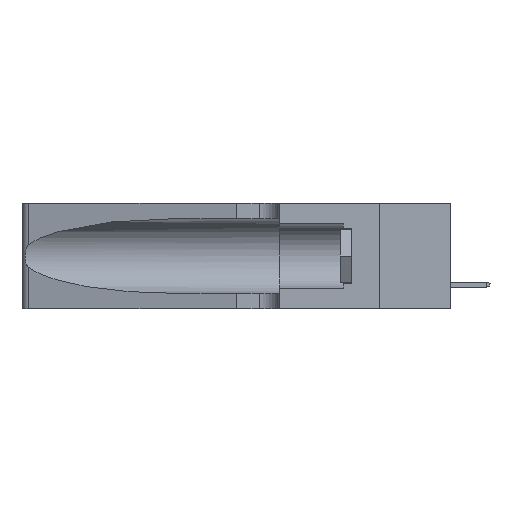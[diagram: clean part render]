
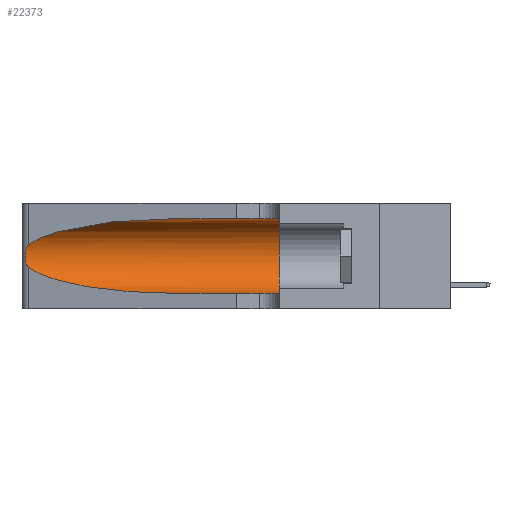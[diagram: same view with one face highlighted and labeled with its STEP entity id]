
A CAD part, left-side view. The second image highlights one B-rep face of the part: STEP entity #22373.
In plain terms, the highlighted cylindrical face has radius 3.308 mm (diameter 6.617 mm), a partial arc.
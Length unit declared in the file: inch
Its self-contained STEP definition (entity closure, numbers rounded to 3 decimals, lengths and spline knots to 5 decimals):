
#98 = VERTEX_POINT ( 'NONE', #26784 ) ;
#1078 = CARTESIAN_POINT ( 'NONE',  ( 0.18966, 0.96281, 0.31525 ) ) ;
#1134 = EDGE_CURVE ( 'NONE', #26663, #29288, #25005, .T. ) ;
#1286 = CARTESIAN_POINT ( 'NONE',  ( 0.26075, 1.23896, 0.19203 ) ) ;
#1718 = CARTESIAN_POINT ( 'NONE',  ( 0.1305, 1.61858, 0.31525 ) ) ;
#2033 =( BOUNDED_CURVE ( )  B_SPLINE_CURVE ( 3, ( #23238, #18377, #27946, #6050 ),
 .UNSPECIFIED., .F., .T. ) 
 B_SPLINE_CURVE_WITH_KNOTS ( ( 4, 4 ),
 ( 3.44316, 4.71239 ),
 .UNSPECIFIED. ) 
 CURVE ( )  GEOMETRIC_REPRESENTATION_ITEM ( )  RATIONAL_B_SPLINE_CURVE ( ( 1., 0.87, 0.87, 1. ) ) 
 REPRESENTATION_ITEM ( '' )  );
#2767 = ORIENTED_EDGE ( 'NONE', *, *, #27312, .F. ) ;
#2822 = CARTESIAN_POINT ( 'NONE',  ( 0.25487, 1.22718, 0.22369 ) ) ;
#3303 = DIRECTION ( 'NONE',  ( 0., 0., -1. ) ) ;
#3975 = DIRECTION ( 'NONE',  ( 0., -1., 0. ) ) ;
#4300 = CARTESIAN_POINT ( 'NONE',  ( 0.25487, 1.22718, 0.14631 ) ) ;
#5276 = CARTESIAN_POINT ( 'NONE',  ( 0.1305, 0.72297, 0.31525 ) ) ;
#5601 = CARTESIAN_POINT ( 'NONE',  ( 0.2373, 1.15595, 0.28018 ) ) ;
#5803 = CARTESIAN_POINT ( 'NONE',  ( 0.25487, 1.22718, 0.14631 ) ) ;
#6050 = CARTESIAN_POINT ( 'NONE',  ( 0.1305, 0.72297, 0.05475 ) ) ;
#6210 = DIRECTION ( 'NONE',  ( 0., 1., 0. ) ) ;
#7992 = DIRECTION ( 'NONE',  ( 0., -1., 0. ) ) ;
#8379 = VERTEX_POINT ( 'NONE', #13891 ) ;
#8678 = AXIS2_PLACEMENT_3D ( 'NONE', #25827, #6210, #30524 ) ;
#8873 = CARTESIAN_POINT ( 'NONE',  ( 0.26017, 1.23833, 0.17102 ) ) ;
#8969 = B_SPLINE_CURVE_WITH_KNOTS ( 'NONE', 3,
 ( #18126, #16009, #21191, #13913, #11004, #18280, #1286, #16162, #8873, #23297, #18605, #18762, #11482, #5803 ),
 .UNSPECIFIED., .F., .F.,
 ( 4, 2, 2, 2, 2, 2, 4 ),
 ( 0., 0.00027, 0.00053, 0.00107, 0.0016, 0.00187, 0.00214 ),
 .UNSPECIFIED. ) ;
#9220 = CIRCLE ( 'NONE', #8678, 0.13025 ) ;
#9975 = AXIS2_PLACEMENT_3D ( 'NONE', #25477, #7992, #3303 ) ;
#10598 = FACE_OUTER_BOUND ( 'NONE', #27418, .T. ) ;
#11004 = CARTESIAN_POINT ( 'NONE',  ( 0.25854, 1.2359, 0.20912 ) ) ;
#11482 = CARTESIAN_POINT ( 'NONE',  ( 0.25555, 1.22993, 0.14849 ) ) ;
#11602 = DIRECTION ( 'NONE',  ( 0., -1., 0. ) ) ;
#11761 = LINE ( 'NONE', #1718, #24561 ) ;
#13891 = CARTESIAN_POINT ( 'NONE',  ( 0.1305, 0.35, 0.05475 ) ) ;
#13913 = CARTESIAN_POINT ( 'NONE',  ( 0.25787, 1.23484, 0.2124 ) ) ;
#15491 = CARTESIAN_POINT ( 'NONE',  ( 0.25487, 1.22718, 0.22369 ) ) ;
#15577 = EDGE_CURVE ( 'NONE', #98, #8379, #9220, .T. ) ;
#16009 = CARTESIAN_POINT ( 'NONE',  ( 0.25555, 1.22994, 0.2215 ) ) ;
#16162 = CARTESIAN_POINT ( 'NONE',  ( 0.26075, 1.23896, 0.178 ) ) ;
#16557 = ORIENTED_EDGE ( 'NONE', *, *, #23697, .T. ) ;
#18126 = CARTESIAN_POINT ( 'NONE',  ( 0.25487, 1.22718, 0.22369 ) ) ;
#18280 = CARTESIAN_POINT ( 'NONE',  ( 0.26018, 1.23835, 0.19895 ) ) ;
#18377 = CARTESIAN_POINT ( 'NONE',  ( 0.2373, 1.15595, 0.08982 ) ) ;
#18458 = EDGE_CURVE ( 'NONE', #26011, #31255, #2033, .T. ) ;
#18605 = CARTESIAN_POINT ( 'NONE',  ( 0.25789, 1.23486, 0.15765 ) ) ;
#18762 = CARTESIAN_POINT ( 'NONE',  ( 0.25639, 1.23186, 0.15144 ) ) ;
#19315 = CARTESIAN_POINT ( 'NONE',  ( 0.1305, 0.72297, 0.31525 ) ) ;
#20826 = CARTESIAN_POINT ( 'NONE',  ( 0.1305, 1.61858, 0.05475 ) ) ;
#21191 = CARTESIAN_POINT ( 'NONE',  ( 0.25639, 1.23184, 0.21858 ) ) ;
#22373 = ADVANCED_FACE ( 'NONE', ( #10598 ), #30811, .F. ) ;
#23238 = CARTESIAN_POINT ( 'NONE',  ( 0.25487, 1.22718, 0.14631 ) ) ;
#23297 = CARTESIAN_POINT ( 'NONE',  ( 0.25856, 1.23593, 0.16098 ) ) ;
#23697 = EDGE_CURVE ( 'NONE', #31255, #8379, #26157, .T. ) ;
#24561 = VECTOR ( 'NONE', #11602, 39.37008 ) ;
#25005 =( BOUNDED_CURVE ( )  B_SPLINE_CURVE ( 3, ( #5276, #1078, #5601, #15491 ),
 .UNSPECIFIED., .F., .T. ) 
 B_SPLINE_CURVE_WITH_KNOTS ( ( 4, 4 ),
 ( 1.5708, 2.84003 ),
 .UNSPECIFIED. ) 
 CURVE ( )  GEOMETRIC_REPRESENTATION_ITEM ( )  RATIONAL_B_SPLINE_CURVE ( ( 1., 0.87, 0.87, 1. ) ) 
 REPRESENTATION_ITEM ( '' )  );
#25477 = CARTESIAN_POINT ( 'NONE',  ( 0.1305, 1.61858, 0.185 ) ) ;
#25827 = CARTESIAN_POINT ( 'NONE',  ( 0.1305, 0.35, 0.185 ) ) ;
#25940 = ORIENTED_EDGE ( 'NONE', *, *, #1134, .T. ) ;
#26011 = VERTEX_POINT ( 'NONE', #4300 ) ;
#26157 = LINE ( 'NONE', #20826, #29633 ) ;
#26663 = VERTEX_POINT ( 'NONE', #19315 ) ;
#26784 = CARTESIAN_POINT ( 'NONE',  ( 0.1305, 0.35, 0.31525 ) ) ;
#27195 = CARTESIAN_POINT ( 'NONE',  ( 0.1305, 0.72297, 0.05475 ) ) ;
#27312 = EDGE_CURVE ( 'NONE', #26663, #98, #11761, .T. ) ;
#27418 = EDGE_LOOP ( 'NONE', ( #25940, #31751, #28858, #16557, #31443, #2767 ) ) ;
#27946 = CARTESIAN_POINT ( 'NONE',  ( 0.18966, 0.96281, 0.05475 ) ) ;
#28858 = ORIENTED_EDGE ( 'NONE', *, *, #18458, .T. ) ;
#29288 = VERTEX_POINT ( 'NONE', #2822 ) ;
#29633 = VECTOR ( 'NONE', #3975, 39.37008 ) ;
#30524 = DIRECTION ( 'NONE',  ( 0., 0., 1. ) ) ;
#30811 = CYLINDRICAL_SURFACE ( 'NONE', #9975, 0.13025 ) ;
#31255 = VERTEX_POINT ( 'NONE', #27195 ) ;
#31443 = ORIENTED_EDGE ( 'NONE', *, *, #15577, .F. ) ;
#31477 = EDGE_CURVE ( 'NONE', #29288, #26011, #8969, .T. ) ;
#31751 = ORIENTED_EDGE ( 'NONE', *, *, #31477, .T. ) ;
